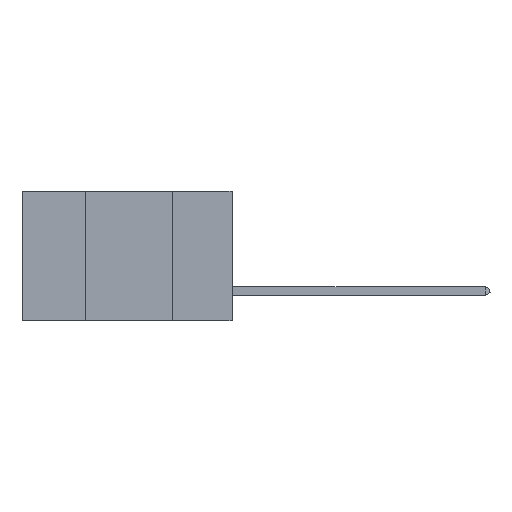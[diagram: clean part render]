
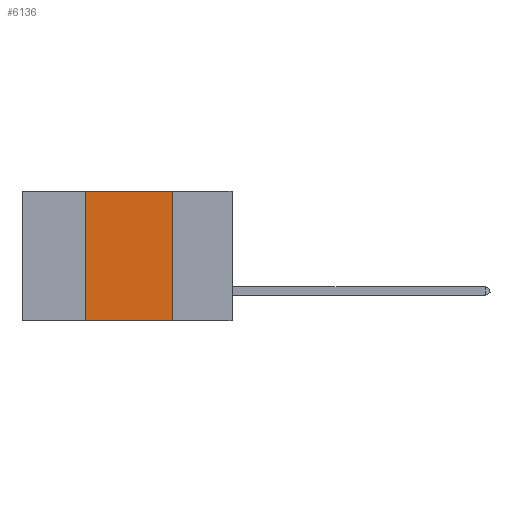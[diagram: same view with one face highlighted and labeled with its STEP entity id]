
A CAD part, left-side view. The second image highlights one B-rep face of the part: STEP entity #6136.
In plain terms, the highlighted planar face has unit normal (-1, 0, 0).
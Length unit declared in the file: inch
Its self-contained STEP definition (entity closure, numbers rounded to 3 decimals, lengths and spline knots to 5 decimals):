
#82 = DIRECTION ( 'NONE',  ( 1., 0., 0. ) ) ;
#101 = LINE ( 'NONE', #5164, #18313 ) ;
#251 = ORIENTED_EDGE ( 'NONE', *, *, #16388, .F. ) ;
#1385 = LINE ( 'NONE', #14603, #9277 ) ;
#1501 = DIRECTION ( 'NONE',  ( 0., 0., -1. ) ) ;
#2018 = EDGE_CURVE ( 'NONE', #17052, #5415, #1385, .T. ) ;
#2064 = EDGE_CURVE ( 'NONE', #7668, #6361, #17063, .T. ) ;
#2298 = EDGE_LOOP ( 'NONE', ( #17627, #18277, #251, #2358 ) ) ;
#2358 = ORIENTED_EDGE ( 'NONE', *, *, #2018, .T. ) ;
#2581 = CARTESIAN_POINT ( 'NONE',  ( 0., 0.17, -0.37 ) ) ;
#5164 = CARTESIAN_POINT ( 'NONE',  ( 0., 0.42, 0. ) ) ;
#5415 = VERTEX_POINT ( 'NONE', #2581 ) ;
#6136 = ADVANCED_FACE ( 'NONE', ( #15824 ), #15860, .F. ) ;
#6361 = VERTEX_POINT ( 'NONE', #12913 ) ;
#6698 = CARTESIAN_POINT ( 'NONE',  ( 0., 0.42, 0. ) ) ;
#7668 = VERTEX_POINT ( 'NONE', #6698 ) ;
#8063 = VECTOR ( 'NONE', #9879, 39.37008 ) ;
#9277 = VECTOR ( 'NONE', #17331, 39.37008 ) ;
#9879 = DIRECTION ( 'NONE',  ( 0., 0., -1. ) ) ;
#9988 = CARTESIAN_POINT ( 'NONE',  ( 0., 0.17, 0. ) ) ;
#12913 = CARTESIAN_POINT ( 'NONE',  ( 0., 0.17, 0. ) ) ;
#13409 = CARTESIAN_POINT ( 'NONE',  ( 0., 0.6, 0. ) ) ;
#13750 = VECTOR ( 'NONE', #14860, 39.37008 ) ;
#14603 = CARTESIAN_POINT ( 'NONE',  ( 0., 0.6, -0.37 ) ) ;
#14860 = DIRECTION ( 'NONE',  ( 0., -1., 0. ) ) ;
#15824 = FACE_OUTER_BOUND ( 'NONE', #2298, .T. ) ;
#15860 = PLANE ( 'NONE',  #18047 ) ;
#16388 = EDGE_CURVE ( 'NONE', #17052, #7668, #101, .T. ) ;
#17006 = LINE ( 'NONE', #9988, #8063 ) ;
#17031 = CARTESIAN_POINT ( 'NONE',  ( 0., 0.42, -0.37 ) ) ;
#17052 = VERTEX_POINT ( 'NONE', #17031 ) ;
#17063 = LINE ( 'NONE', #13409, #13750 ) ;
#17331 = DIRECTION ( 'NONE',  ( 0., -1., 0. ) ) ;
#17405 = CARTESIAN_POINT ( 'NONE',  ( 0., 0.6, 0. ) ) ;
#17627 = ORIENTED_EDGE ( 'NONE', *, *, #18291, .F. ) ;
#18047 = AXIS2_PLACEMENT_3D ( 'NONE', #17405, #82, #1501 ) ;
#18277 = ORIENTED_EDGE ( 'NONE', *, *, #2064, .F. ) ;
#18291 = EDGE_CURVE ( 'NONE', #6361, #5415, #17006, .T. ) ;
#18313 = VECTOR ( 'NONE', #18334, 39.37008 ) ;
#18334 = DIRECTION ( 'NONE',  ( 0., 0., 1. ) ) ;
